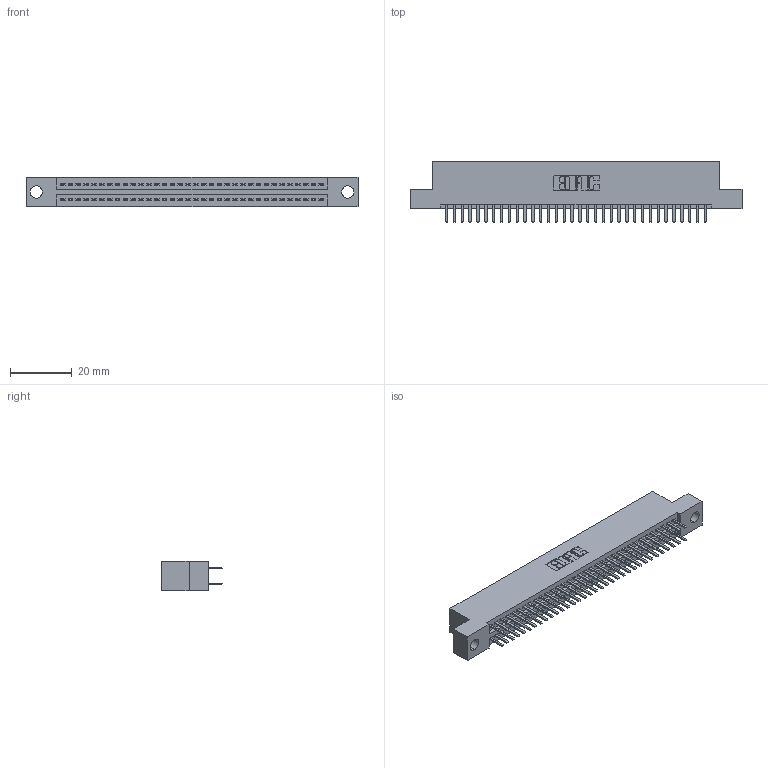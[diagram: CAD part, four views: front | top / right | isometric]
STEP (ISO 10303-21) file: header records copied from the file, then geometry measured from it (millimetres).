
FILE_DESCRIPTION (( 'STEP AP203' ), '1' );
FILE_NAME ('395-068-520-204.STEP', '2018-11-25T12:05:37', ( '' ), ( '' ), 'SwSTEP 2.0', 'SolidWorks 2016', '' );
FILE_SCHEMA (( 'CONFIG_CONTROL_DESIGN' ));
Length unit declared in the file: inch
Products named in the file (3): 345-292-001_345-293-120; 345 Part_Flush Mounting Lugs - 0.156 Dia-TH; 395-068-520-204
Assembly tree (69 placements, depth 2):
  395-068-520-204
    345 Part_Flush Mounting Lugs - 0.156 Dia-TH
    345-292-001_345-293-120  x68
Bounding box: 107.57 x 19.68 x 9.4 mm (x, y, z)
Volume: 10257.4 mm3; surface area: 14758.7 mm2
Topology: 69 solids, 69 shells, 3798 faces, 11017 edges, 7162 vertices
Faces by surface type: plane 2460, cylinder 1338
Entity records: 27871 total; most frequent: CARTESIAN_POINT 4692, ORIENTED_EDGE 4614, DIRECTION 4135, EDGE_CURVE 2307, VECTOR 2035, LINE 2035, VERTEX_POINT 1534, AXIS2_PLACEMENT_3D 1050
